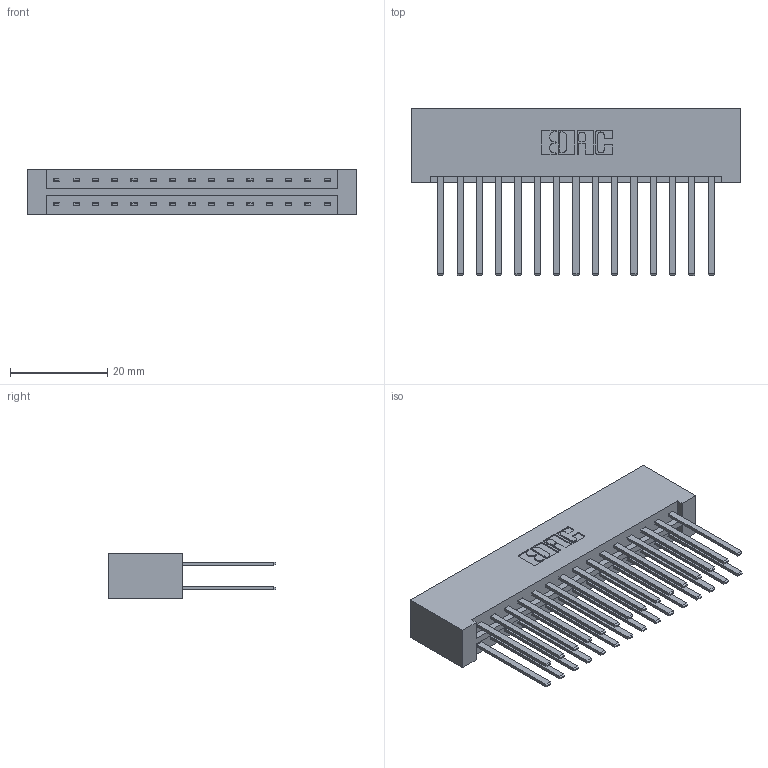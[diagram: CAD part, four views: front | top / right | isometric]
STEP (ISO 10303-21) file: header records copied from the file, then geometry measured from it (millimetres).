
FILE_DESCRIPTION (( 'STEP AP203' ), '1' );
FILE_NAME ('833-030-544-201.STEP', '2020-06-02T13:39:39', ( '' ), ( '' ), 'SwSTEP 2.0', 'SolidWorks 2020', '' );
FILE_SCHEMA (( 'CONFIG_CONTROL_DESIGN' ));
Length unit declared in the file: inch
Products named in the file (3): 833 Part_Lugless; 345-292-001_345-293-144; 833-030-544-201
Assembly tree (31 placements, depth 2):
  833-030-544-201
    833 Part_Lugless
    345-292-001_345-293-144  x30
Bounding box: 67.69 x 34.3 x 9.4 mm (x, y, z)
Volume: 7711.1 mm3; surface area: 10204.8 mm2
Topology: 31 solids, 31 shells, 1486 faces, 4397 edges, 2890 vertices
Faces by surface type: plane 1026, cylinder 460
Entity records: 12681 total; most frequent: CARTESIAN_POINT 2130, ORIENTED_EDGE 2066, DIRECTION 1857, EDGE_CURVE 1033, VECTOR 917, LINE 917, VERTEX_POINT 686, AXIS2_PLACEMENT_3D 470
